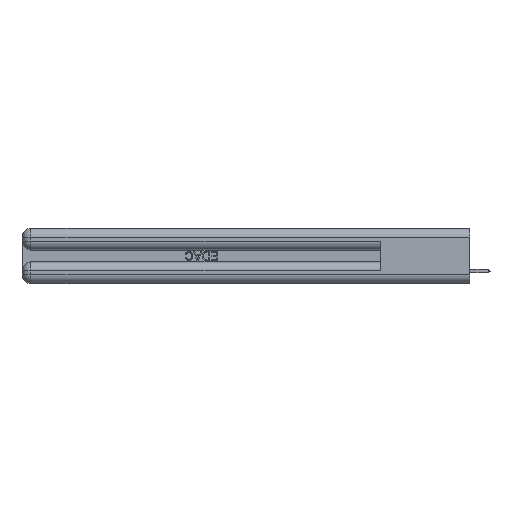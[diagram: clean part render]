
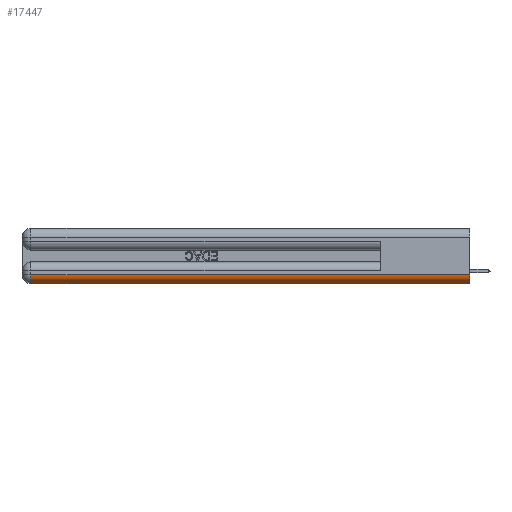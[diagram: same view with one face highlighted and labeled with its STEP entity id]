
A CAD part, left-side view. The second image highlights one B-rep face of the part: STEP entity #17447.
In plain terms, the highlighted cylindrical face has radius 1.524 mm (diameter 3.048 mm), a partial arc.
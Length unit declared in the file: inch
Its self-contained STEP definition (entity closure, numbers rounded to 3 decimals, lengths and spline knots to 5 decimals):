
#1174 = DIRECTION ( 'NONE',  ( 0., 0., 1. ) ) ;
#2772 = LINE ( 'NONE', #25428, #36963 ) ;
#3417 = ORIENTED_EDGE ( 'NONE', *, *, #31034, .F. ) ;
#3546 = EDGE_LOOP ( 'NONE', ( #12644, #3417, #17696, #25210 ) ) ;
#5631 = VECTOR ( 'NONE', #11403, 39.37008 ) ;
#6087 = FACE_OUTER_BOUND ( 'NONE', #3546, .T. ) ;
#6864 = CARTESIAN_POINT ( 'NONE',  ( 0., 0., 0.06 ) ) ;
#7270 = VERTEX_POINT ( 'NONE', #14172 ) ;
#7321 = CIRCLE ( 'NONE', #27573, 0.06 ) ;
#7646 = DIRECTION ( 'NONE',  ( 0., 1., 0. ) ) ;
#8026 = DIRECTION ( 'NONE',  ( 0., 0., 1. ) ) ;
#8630 = DIRECTION ( 'NONE',  ( 0., -1., 0. ) ) ;
#11166 = VERTEX_POINT ( 'NONE', #13609 ) ;
#11315 = EDGE_CURVE ( 'NONE', #27609, #7270, #2772, .T. ) ;
#11403 = DIRECTION ( 'NONE',  ( 0., -1., 0. ) ) ;
#12644 = ORIENTED_EDGE ( 'NONE', *, *, #22659, .F. ) ;
#13609 = CARTESIAN_POINT ( 'NONE',  ( 0., 2.94, 0.06 ) ) ;
#14172 = CARTESIAN_POINT ( 'NONE',  ( 0.06, 2.94, 0. ) ) ;
#15064 = CARTESIAN_POINT ( 'NONE',  ( 0.06, 0., 0.06 ) ) ;
#17447 = ADVANCED_FACE ( 'NONE', ( #6087 ), #31486, .T. ) ;
#17512 = AXIS2_PLACEMENT_3D ( 'NONE', #20163, #19890, #1174 ) ;
#17696 = ORIENTED_EDGE ( 'NONE', *, *, #25695, .F. ) ;
#18561 = AXIS2_PLACEMENT_3D ( 'NONE', #39154, #29896, #8026 ) ;
#19890 = DIRECTION ( 'NONE',  ( 0., 1., 0. ) ) ;
#20163 = CARTESIAN_POINT ( 'NONE',  ( 0.06, 0., 0.06 ) ) ;
#22659 = EDGE_CURVE ( 'NONE', #30782, #27609, #7321, .T. ) ;
#25210 = ORIENTED_EDGE ( 'NONE', *, *, #11315, .F. ) ;
#25428 = CARTESIAN_POINT ( 'NONE',  ( 0.06, 3., 0. ) ) ;
#25695 = EDGE_CURVE ( 'NONE', #7270, #11166, #36912, .T. ) ;
#27209 = LINE ( 'NONE', #32293, #5631 ) ;
#27573 = AXIS2_PLACEMENT_3D ( 'NONE', #15064, #8630, #30767 ) ;
#27609 = VERTEX_POINT ( 'NONE', #31793 ) ;
#29896 = DIRECTION ( 'NONE',  ( 0., 1., 0. ) ) ;
#30767 = DIRECTION ( 'NONE',  ( 0., 0., 1. ) ) ;
#30782 = VERTEX_POINT ( 'NONE', #6864 ) ;
#31034 = EDGE_CURVE ( 'NONE', #11166, #30782, #27209, .T. ) ;
#31486 = CYLINDRICAL_SURFACE ( 'NONE', #17512, 0.06 ) ;
#31793 = CARTESIAN_POINT ( 'NONE',  ( 0.06, 0., 0. ) ) ;
#32293 = CARTESIAN_POINT ( 'NONE',  ( 0., 0., 0.06 ) ) ;
#36912 = CIRCLE ( 'NONE', #18561, 0.06 ) ;
#36963 = VECTOR ( 'NONE', #7646, 39.37008 ) ;
#39154 = CARTESIAN_POINT ( 'NONE',  ( 0.06, 2.94, 0.06 ) ) ;
